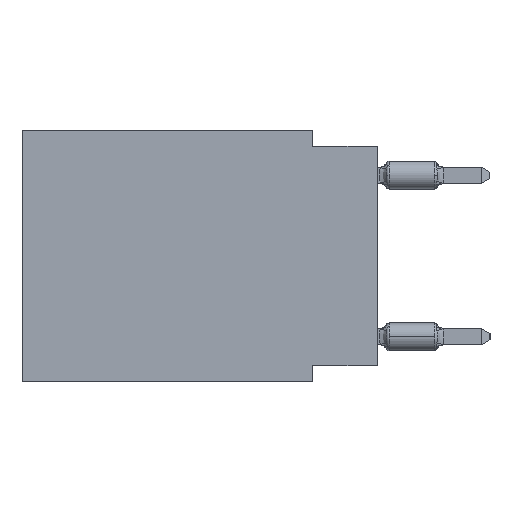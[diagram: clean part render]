
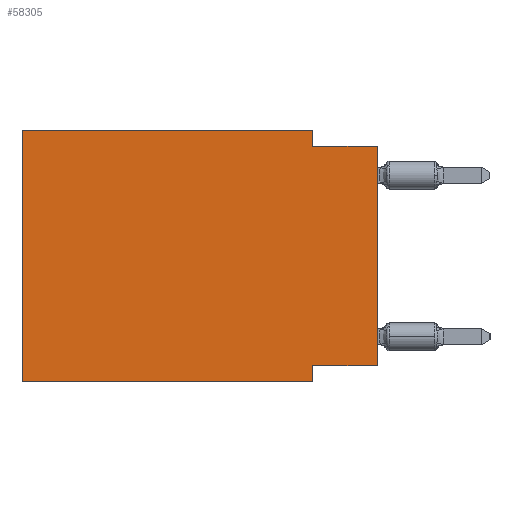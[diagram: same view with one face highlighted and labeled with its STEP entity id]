
A CAD part, left-side view. The second image highlights one B-rep face of the part: STEP entity #58305.
In plain terms, the highlighted planar face has unit normal (-1, 0, 0).
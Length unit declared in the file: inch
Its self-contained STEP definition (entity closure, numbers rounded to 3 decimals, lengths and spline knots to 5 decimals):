
#255 = CARTESIAN_POINT ( 'NONE',  ( 0., 0.55, 0. ) ) ;
#1695 = EDGE_CURVE ( 'NONE', #18253, #27148, #14614, .T. ) ;
#2967 = EDGE_CURVE ( 'NONE', #49561, #28828, #65597, .T. ) ;
#3393 = CARTESIAN_POINT ( 'NONE',  ( 0., 0.55, 0. ) ) ;
#3600 = DIRECTION ( 'NONE',  ( 0., 0., -1. ) ) ;
#7366 = LINE ( 'NONE', #58295, #9131 ) ;
#7629 = PLANE ( 'NONE',  #63311 ) ;
#8469 = CARTESIAN_POINT ( 'NONE',  ( 0., 0., -0.365 ) ) ;
#9131 = VECTOR ( 'NONE', #43237, 39.37008 ) ;
#11489 = VECTOR ( 'NONE', #28931, 39.37008 ) ;
#14002 = VECTOR ( 'NONE', #3600, 39.37008 ) ;
#14588 = VERTEX_POINT ( 'NONE', #62804 ) ;
#14614 = LINE ( 'NONE', #50513, #19679 ) ;
#14917 = CARTESIAN_POINT ( 'NONE',  ( 0., 0.1, -0.365 ) ) ;
#16871 = CARTESIAN_POINT ( 'NONE',  ( 0., 0., 0. ) ) ;
#16873 = ORIENTED_EDGE ( 'NONE', *, *, #1695, .F. ) ;
#17150 = ORIENTED_EDGE ( 'NONE', *, *, #27330, .F. ) ;
#18253 = VERTEX_POINT ( 'NONE', #255 ) ;
#18501 = LINE ( 'NONE', #38970, #54299 ) ;
#19679 = VECTOR ( 'NONE', #55882, 39.37008 ) ;
#26431 = VECTOR ( 'NONE', #28918, 39.37008 ) ;
#27148 = VERTEX_POINT ( 'NONE', #36686 ) ;
#27330 = EDGE_CURVE ( 'NONE', #28908, #62719, #32638, .T. ) ;
#28084 = CARTESIAN_POINT ( 'NONE',  ( 0., 0.55, 0. ) ) ;
#28409 = EDGE_CURVE ( 'NONE', #28908, #28828, #47087, .T. ) ;
#28720 = FACE_OUTER_BOUND ( 'NONE', #38577, .T. ) ;
#28828 = VERTEX_POINT ( 'NONE', #47346 ) ;
#28908 = VERTEX_POINT ( 'NONE', #56734 ) ;
#28918 = DIRECTION ( 'NONE',  ( 0., 1., 0. ) ) ;
#28931 = DIRECTION ( 'NONE',  ( 0., 0., 1. ) ) ;
#32638 = LINE ( 'NONE', #8469, #26431 ) ;
#33928 = VERTEX_POINT ( 'NONE', #64975 ) ;
#35968 = EDGE_CURVE ( 'NONE', #14588, #18253, #43970, .T. ) ;
#36415 = EDGE_CURVE ( 'NONE', #27148, #49561, #7366, .T. ) ;
#36686 = CARTESIAN_POINT ( 'NONE',  ( 0., 0.1, 0. ) ) ;
#36955 = VECTOR ( 'NONE', #48653, 39.37008 ) ;
#38577 = EDGE_LOOP ( 'NONE', ( #64502, #63950, #55591, #16873, #64842, #58968, #43696, #17150 ) ) ;
#38970 = CARTESIAN_POINT ( 'NONE',  ( 0., 0.55, -0.39 ) ) ;
#43237 = DIRECTION ( 'NONE',  ( 0., 0., -1. ) ) ;
#43696 = ORIENTED_EDGE ( 'NONE', *, *, #44359, .F. ) ;
#43970 = LINE ( 'NONE', #3393, #36955 ) ;
#44359 = EDGE_CURVE ( 'NONE', #62719, #33928, #49515, .T. ) ;
#47087 = LINE ( 'NONE', #16871, #11489 ) ;
#47346 = CARTESIAN_POINT ( 'NONE',  ( 0., 0., -0.025 ) ) ;
#48653 = DIRECTION ( 'NONE',  ( 0., 0., 1. ) ) ;
#49515 = LINE ( 'NONE', #53558, #14002 ) ;
#49561 = VERTEX_POINT ( 'NONE', #60656 ) ;
#50513 = CARTESIAN_POINT ( 'NONE',  ( 0., 0.55, 0. ) ) ;
#50855 = CARTESIAN_POINT ( 'NONE',  ( 0., 0., -0.025 ) ) ;
#53185 = VECTOR ( 'NONE', #56221, 39.37008 ) ;
#53558 = CARTESIAN_POINT ( 'NONE',  ( 0., 0.1, -0.39 ) ) ;
#54190 = DIRECTION ( 'NONE',  ( 0., 0., -1. ) ) ;
#54299 = VECTOR ( 'NONE', #54705, 39.37008 ) ;
#54705 = DIRECTION ( 'NONE',  ( 0., -1., 0. ) ) ;
#54860 = DIRECTION ( 'NONE',  ( 1., 0., 0. ) ) ;
#55591 = ORIENTED_EDGE ( 'NONE', *, *, #36415, .F. ) ;
#55882 = DIRECTION ( 'NONE',  ( 0., -1., 0. ) ) ;
#56221 = DIRECTION ( 'NONE',  ( 0., -1., 0. ) ) ;
#56734 = CARTESIAN_POINT ( 'NONE',  ( 0., 0., -0.365 ) ) ;
#58295 = CARTESIAN_POINT ( 'NONE',  ( 0., 0.1, 0. ) ) ;
#58305 = ADVANCED_FACE ( 'NONE', ( #28720 ), #7629, .F. ) ;
#58968 = ORIENTED_EDGE ( 'NONE', *, *, #61921, .T. ) ;
#60656 = CARTESIAN_POINT ( 'NONE',  ( 0., 0.1, -0.025 ) ) ;
#61921 = EDGE_CURVE ( 'NONE', #14588, #33928, #18501, .T. ) ;
#62719 = VERTEX_POINT ( 'NONE', #14917 ) ;
#62804 = CARTESIAN_POINT ( 'NONE',  ( 0., 0.55, -0.39 ) ) ;
#63311 = AXIS2_PLACEMENT_3D ( 'NONE', #28084, #54860, #54190 ) ;
#63950 = ORIENTED_EDGE ( 'NONE', *, *, #2967, .F. ) ;
#64502 = ORIENTED_EDGE ( 'NONE', *, *, #28409, .T. ) ;
#64842 = ORIENTED_EDGE ( 'NONE', *, *, #35968, .F. ) ;
#64975 = CARTESIAN_POINT ( 'NONE',  ( 0., 0.1, -0.39 ) ) ;
#65597 = LINE ( 'NONE', #50855, #53185 ) ;
